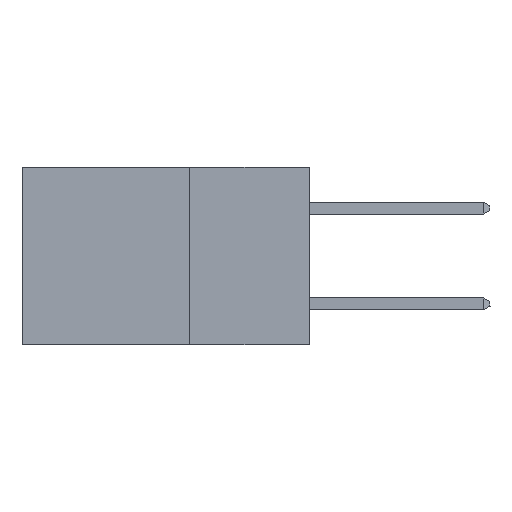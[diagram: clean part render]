
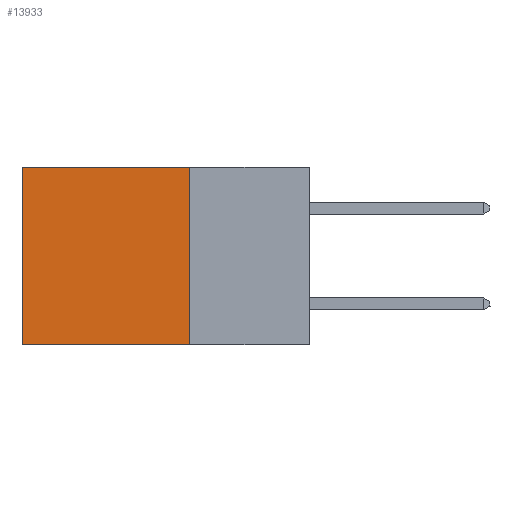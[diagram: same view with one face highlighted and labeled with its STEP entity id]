
A CAD part, left-side view. The second image highlights one B-rep face of the part: STEP entity #13933.
In plain terms, the highlighted planar face has unit normal (-1, 0, 0).
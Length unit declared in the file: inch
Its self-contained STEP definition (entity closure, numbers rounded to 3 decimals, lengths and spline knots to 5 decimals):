
#128 = DIRECTION ( 'NONE',  ( 0., 0., -1. ) ) ;
#224 = VERTEX_POINT ( 'NONE', #14526 ) ;
#988 = CARTESIAN_POINT ( 'NONE',  ( 0.2875, 0.6, 0. ) ) ;
#1242 = EDGE_CURVE ( 'NONE', #14273, #224, #16058, .T. ) ;
#1592 = VECTOR ( 'NONE', #11713, 39.37008 ) ;
#1723 = ORIENTED_EDGE ( 'NONE', *, *, #17887, .F. ) ;
#2323 = DIRECTION ( 'NONE',  ( 0., 1., 0. ) ) ;
#2472 = CARTESIAN_POINT ( 'NONE',  ( 0.2875, 0.6, 0. ) ) ;
#3058 = CARTESIAN_POINT ( 'NONE',  ( 0.2875, 0.25, 0. ) ) ;
#3122 = EDGE_LOOP ( 'NONE', ( #7836, #6229, #1723, #3454 ) ) ;
#3330 = EDGE_CURVE ( 'NONE', #11083, #224, #5860, .T. ) ;
#3454 = ORIENTED_EDGE ( 'NONE', *, *, #7104, .T. ) ;
#3471 = CARTESIAN_POINT ( 'NONE',  ( 0.2875, 0.25, -0.37 ) ) ;
#3505 = VECTOR ( 'NONE', #7176, 39.37008 ) ;
#3615 = LINE ( 'NONE', #8474, #18333 ) ;
#5618 = DIRECTION ( 'NONE',  ( 0., 1., 0. ) ) ;
#5860 = LINE ( 'NONE', #3471, #6339 ) ;
#6229 = ORIENTED_EDGE ( 'NONE', *, *, #3330, .F. ) ;
#6339 = VECTOR ( 'NONE', #5618, 39.37008 ) ;
#7104 = EDGE_CURVE ( 'NONE', #9367, #14273, #3615, .T. ) ;
#7176 = DIRECTION ( 'NONE',  ( 0., 0., -1. ) ) ;
#7493 = CARTESIAN_POINT ( 'NONE',  ( 0.2875, 0.25, -0.37 ) ) ;
#7574 = AXIS2_PLACEMENT_3D ( 'NONE', #18733, #9486, #128 ) ;
#7836 = ORIENTED_EDGE ( 'NONE', *, *, #1242, .T. ) ;
#8474 = CARTESIAN_POINT ( 'NONE',  ( 0.2875, 0.25, 0. ) ) ;
#9367 = VERTEX_POINT ( 'NONE', #3058 ) ;
#9486 = DIRECTION ( 'NONE',  ( 1., 0., 0. ) ) ;
#10817 = PLANE ( 'NONE',  #7574 ) ;
#11083 = VERTEX_POINT ( 'NONE', #7493 ) ;
#11713 = DIRECTION ( 'NONE',  ( 0., 0., -1. ) ) ;
#13899 = LINE ( 'NONE', #14801, #1592 ) ;
#13933 = ADVANCED_FACE ( 'NONE', ( #19497 ), #10817, .F. ) ;
#14273 = VERTEX_POINT ( 'NONE', #988 ) ;
#14526 = CARTESIAN_POINT ( 'NONE',  ( 0.2875, 0.6, -0.37 ) ) ;
#14801 = CARTESIAN_POINT ( 'NONE',  ( 0.2875, 0.25, 0. ) ) ;
#16058 = LINE ( 'NONE', #2472, #3505 ) ;
#17887 = EDGE_CURVE ( 'NONE', #9367, #11083, #13899, .T. ) ;
#18333 = VECTOR ( 'NONE', #2323, 39.37008 ) ;
#18733 = CARTESIAN_POINT ( 'NONE',  ( 0.2875, 0.25, 0. ) ) ;
#19497 = FACE_OUTER_BOUND ( 'NONE', #3122, .T. ) ;
